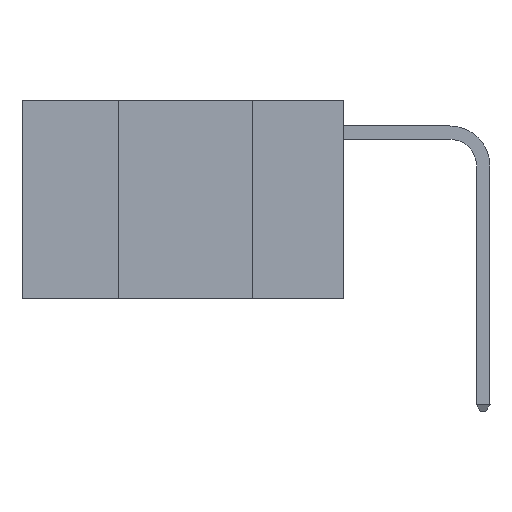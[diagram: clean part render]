
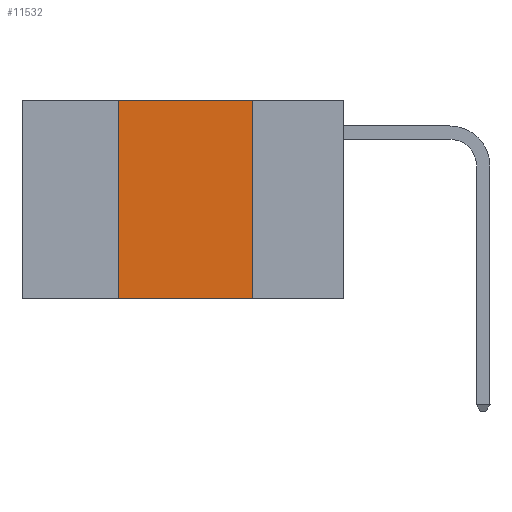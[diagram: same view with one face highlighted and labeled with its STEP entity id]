
A CAD part, left-side view. The second image highlights one B-rep face of the part: STEP entity #11532.
In plain terms, the highlighted planar face has unit normal (-1, 0, 0).
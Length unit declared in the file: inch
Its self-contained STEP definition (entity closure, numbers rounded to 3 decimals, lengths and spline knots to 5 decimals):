
#378 = EDGE_CURVE ( 'NONE', #4082, #5696, #12859, .T. ) ;
#826 = EDGE_CURVE ( 'NONE', #4695, #4082, #9554, .T. ) ;
#1334 = EDGE_CURVE ( 'NONE', #12304, #4695, #6952, .T. ) ;
#1587 = CARTESIAN_POINT ( 'NONE',  ( 0., 0.17, -0.37 ) ) ;
#2043 = ORIENTED_EDGE ( 'NONE', *, *, #378, .F. ) ;
#2064 = ORIENTED_EDGE ( 'NONE', *, *, #826, .F. ) ;
#2140 = ORIENTED_EDGE ( 'NONE', *, *, #1334, .F. ) ;
#2159 = ORIENTED_EDGE ( 'NONE', *, *, #7289, .T. ) ;
#2328 = FACE_OUTER_BOUND ( 'NONE', #16166, .T. ) ;
#3159 = DIRECTION ( 'NONE',  ( 0., -1., 0. ) ) ;
#3241 = CARTESIAN_POINT ( 'NONE',  ( 0., 0.6, -0.37 ) ) ;
#4082 = VERTEX_POINT ( 'NONE', #13946 ) ;
#4695 = VERTEX_POINT ( 'NONE', #5128 ) ;
#4925 = PLANE ( 'NONE',  #11091 ) ;
#5023 = VECTOR ( 'NONE', #3159, 39.37008 ) ;
#5058 = LINE ( 'NONE', #3241, #5023 ) ;
#5128 = CARTESIAN_POINT ( 'NONE',  ( 0., 0.42, 0. ) ) ;
#5696 = VERTEX_POINT ( 'NONE', #1587 ) ;
#6222 = DIRECTION ( 'NONE',  ( 0., 0., -1. ) ) ;
#6921 = VECTOR ( 'NONE', #12946, 39.37008 ) ;
#6952 = LINE ( 'NONE', #16212, #6921 ) ;
#7002 = CARTESIAN_POINT ( 'NONE',  ( 0., 0.6, 0. ) ) ;
#7289 = EDGE_CURVE ( 'NONE', #12304, #5696, #5058, .T. ) ;
#7560 = DIRECTION ( 'NONE',  ( 0., -1., 0. ) ) ;
#7920 = CARTESIAN_POINT ( 'NONE',  ( 0., 0.42, -0.37 ) ) ;
#8262 = DIRECTION ( 'NONE',  ( 0., 0., -1. ) ) ;
#8795 = CARTESIAN_POINT ( 'NONE',  ( 0., 0.6, 0. ) ) ;
#9431 = VECTOR ( 'NONE', #7560, 39.37008 ) ;
#9554 = LINE ( 'NONE', #7002, #9431 ) ;
#10991 = CARTESIAN_POINT ( 'NONE',  ( 0., 0.17, 0. ) ) ;
#11091 = AXIS2_PLACEMENT_3D ( 'NONE', #8795, #13860, #6222 ) ;
#11532 = ADVANCED_FACE ( 'NONE', ( #2328 ), #4925, .F. ) ;
#12304 = VERTEX_POINT ( 'NONE', #7920 ) ;
#12846 = VECTOR ( 'NONE', #8262, 39.37008 ) ;
#12859 = LINE ( 'NONE', #10991, #12846 ) ;
#12946 = DIRECTION ( 'NONE',  ( 0., 0., 1. ) ) ;
#13860 = DIRECTION ( 'NONE',  ( 1., 0., 0. ) ) ;
#13946 = CARTESIAN_POINT ( 'NONE',  ( 0., 0.17, 0. ) ) ;
#16166 = EDGE_LOOP ( 'NONE', ( #2043, #2064, #2140, #2159 ) ) ;
#16212 = CARTESIAN_POINT ( 'NONE',  ( 0., 0.42, 0. ) ) ;
